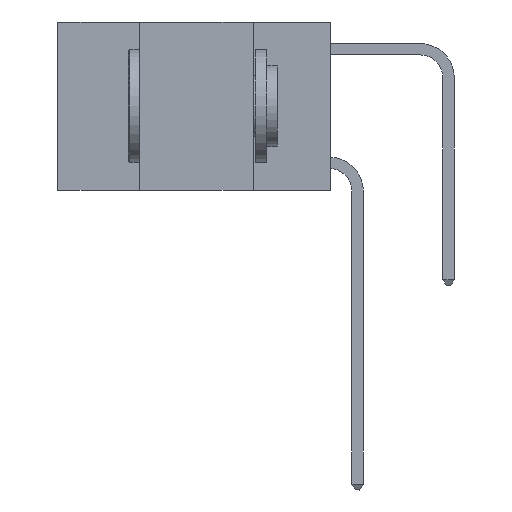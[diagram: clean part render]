
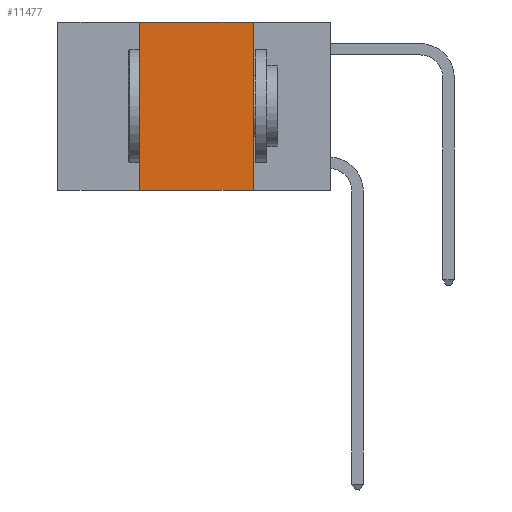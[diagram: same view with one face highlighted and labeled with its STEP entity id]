
A CAD part, left-side view. The second image highlights one B-rep face of the part: STEP entity #11477.
In plain terms, the highlighted planar face has unit normal (-1, 0, 0).
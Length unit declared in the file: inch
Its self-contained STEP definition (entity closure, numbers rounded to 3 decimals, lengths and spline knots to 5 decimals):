
#1496 = LINE ( 'NONE', #12148, #15440 ) ;
#1727 = CARTESIAN_POINT ( 'NONE',  ( 0., 0.17, 0. ) ) ;
#3051 = DIRECTION ( 'NONE',  ( 0., -1., 0. ) ) ;
#3663 = DIRECTION ( 'NONE',  ( 1., 0., 0. ) ) ;
#4224 = VERTEX_POINT ( 'NONE', #6523 ) ;
#4919 = VERTEX_POINT ( 'NONE', #8314 ) ;
#5961 = VECTOR ( 'NONE', #3051, 39.37008 ) ;
#6178 = DIRECTION ( 'NONE',  ( 0., 0., 1. ) ) ;
#6523 = CARTESIAN_POINT ( 'NONE',  ( 0., 0.42, -0.37 ) ) ;
#6549 = CARTESIAN_POINT ( 'NONE',  ( 0., 0.6, 0. ) ) ;
#6864 = DIRECTION ( 'NONE',  ( 0., -1., 0. ) ) ;
#7152 = DIRECTION ( 'NONE',  ( 0., 0., -1. ) ) ;
#7436 = ORIENTED_EDGE ( 'NONE', *, *, #11144, .T. ) ;
#7567 = ORIENTED_EDGE ( 'NONE', *, *, #14956, .F. ) ;
#7759 = VECTOR ( 'NONE', #6178, 39.37008 ) ;
#8314 = CARTESIAN_POINT ( 'NONE',  ( 0., 0.17, -0.37 ) ) ;
#8773 = ORIENTED_EDGE ( 'NONE', *, *, #17571, .F. ) ;
#9069 = CARTESIAN_POINT ( 'NONE',  ( 0., 0.42, 0. ) ) ;
#9341 = PLANE ( 'NONE',  #13919 ) ;
#9809 = ORIENTED_EDGE ( 'NONE', *, *, #14677, .F. ) ;
#10090 = CARTESIAN_POINT ( 'NONE',  ( 0., 0.6, -0.37 ) ) ;
#11144 = EDGE_CURVE ( 'NONE', #4224, #4919, #12798, .T. ) ;
#11145 = CARTESIAN_POINT ( 'NONE',  ( 0., 0.17, 0. ) ) ;
#11477 = ADVANCED_FACE ( 'NONE', ( #15182 ), #9341, .F. ) ;
#11561 = CARTESIAN_POINT ( 'NONE',  ( 0., 0.42, 0. ) ) ;
#12148 = CARTESIAN_POINT ( 'NONE',  ( 0., 0.6, 0. ) ) ;
#12563 = VERTEX_POINT ( 'NONE', #11561 ) ;
#12745 = LINE ( 'NONE', #11145, #15553 ) ;
#12798 = LINE ( 'NONE', #10090, #5961 ) ;
#13351 = DIRECTION ( 'NONE',  ( 0., 0., -1. ) ) ;
#13409 = VERTEX_POINT ( 'NONE', #1727 ) ;
#13919 = AXIS2_PLACEMENT_3D ( 'NONE', #6549, #3663, #13351 ) ;
#14223 = EDGE_LOOP ( 'NONE', ( #9809, #8773, #7567, #7436 ) ) ;
#14677 = EDGE_CURVE ( 'NONE', #13409, #4919, #12745, .T. ) ;
#14956 = EDGE_CURVE ( 'NONE', #4224, #12563, #15775, .T. ) ;
#15182 = FACE_OUTER_BOUND ( 'NONE', #14223, .T. ) ;
#15440 = VECTOR ( 'NONE', #6864, 39.37008 ) ;
#15553 = VECTOR ( 'NONE', #7152, 39.37008 ) ;
#15775 = LINE ( 'NONE', #9069, #7759 ) ;
#17571 = EDGE_CURVE ( 'NONE', #12563, #13409, #1496, .T. ) ;
